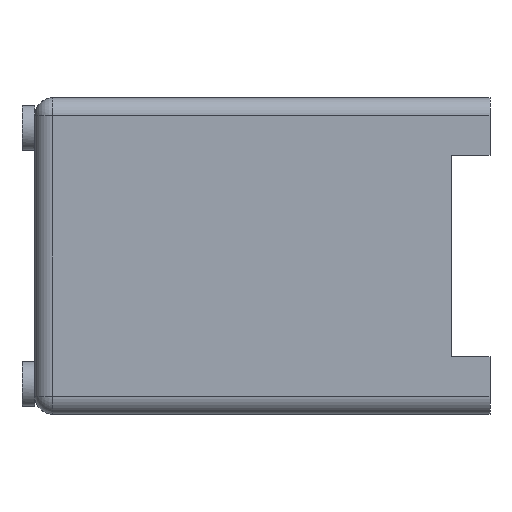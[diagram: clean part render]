
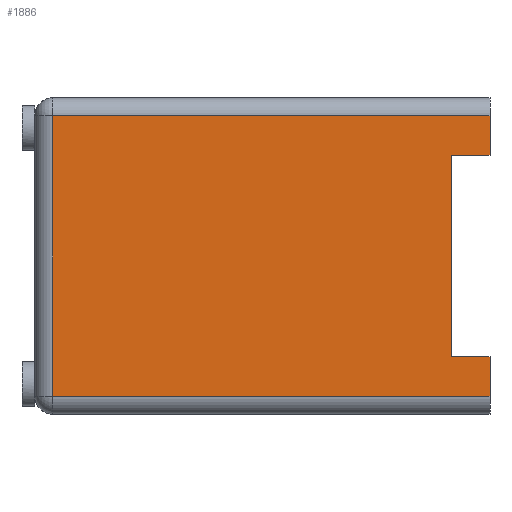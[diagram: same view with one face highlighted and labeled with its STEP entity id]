
A CAD part, left-side view. The second image highlights one B-rep face of the part: STEP entity #1886.
In plain terms, the highlighted planar face has unit normal (-1, 0, 0).
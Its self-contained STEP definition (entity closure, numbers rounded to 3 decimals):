
#4 = EDGE_CURVE ( 'NONE', #798, #2112, #1876, .T. ) ;
#59 = DIRECTION ( 'NONE',  ( 0., 0., 1. ) ) ;
#72 = ORIENTED_EDGE ( 'NONE', *, *, #1344, .T. ) ;
#96 = DIRECTION ( 'NONE',  ( -1., 0., 0. ) ) ;
#103 = CARTESIAN_POINT ( 'NONE',  ( 0., 0., -29.566 ) ) ;
#123 = DIRECTION ( 'NONE',  ( 0., 0., -1. ) ) ;
#158 = ORIENTED_EDGE ( 'NONE', *, *, #684, .T. ) ;
#226 = EDGE_CURVE ( 'NONE', #2142, #892, #342, .T. ) ;
#231 = CARTESIAN_POINT ( 'NONE',  ( 0., 0., -5.69 ) ) ;
#252 = LINE ( 'NONE', #1447, #1040 ) ;
#303 = ORIENTED_EDGE ( 'NONE', *, *, #226, .T. ) ;
#342 = LINE ( 'NONE', #858, #1120 ) ;
#353 = CARTESIAN_POINT ( 'NONE',  ( 0., 43.307, -29.566 ) ) ;
#359 = VERTEX_POINT ( 'NONE', #1167 ) ;
#436 = LINE ( 'NONE', #103, #1429 ) ;
#439 = FACE_OUTER_BOUND ( 'NONE', #701, .T. ) ;
#496 = CARTESIAN_POINT ( 'NONE',  ( 0., 3.81, -5.69 ) ) ;
#515 = DIRECTION ( 'NONE',  ( 0., 0., -1. ) ) ;
#518 = DIRECTION ( 'NONE',  ( 0., 1., 0. ) ) ;
#522 = CARTESIAN_POINT ( 'NONE',  ( 0., 0., -1.778 ) ) ;
#523 = VERTEX_POINT ( 'NONE', #648 ) ;
#631 = DIRECTION ( 'NONE',  ( 0., -1., 0. ) ) ;
#648 = CARTESIAN_POINT ( 'NONE',  ( 0., 0., -29.566 ) ) ;
#657 = EDGE_CURVE ( 'NONE', #1783, #798, #669, .T. ) ;
#659 = CARTESIAN_POINT ( 'NONE',  ( 0., 0., -31.344 ) ) ;
#669 = LINE ( 'NONE', #496, #1096 ) ;
#679 = DIRECTION ( 'NONE',  ( 0., 0., 1. ) ) ;
#684 = EDGE_CURVE ( 'NONE', #523, #359, #1039, .T. ) ;
#698 = DIRECTION ( 'NONE',  ( 0., 1., 0. ) ) ;
#701 = EDGE_LOOP ( 'NONE', ( #2116, #303, #1740, #72, #158, #1464, #1935, #825 ) ) ;
#784 = VECTOR ( 'NONE', #59, 1000. ) ;
#798 = VERTEX_POINT ( 'NONE', #2208 ) ;
#825 = ORIENTED_EDGE ( 'NONE', *, *, #657, .F. ) ;
#854 = EDGE_CURVE ( 'NONE', #892, #2178, #2091, .T. ) ;
#858 = CARTESIAN_POINT ( 'NONE',  ( 0., 45.085, -1.778 ) ) ;
#873 = CARTESIAN_POINT ( 'NONE',  ( 0., 43.307, -1.778 ) ) ;
#892 = VERTEX_POINT ( 'NONE', #873 ) ;
#947 = DIRECTION ( 'NONE',  ( 0., 0., 1. ) ) ;
#989 = LINE ( 'NONE', #1873, #784 ) ;
#1002 = CARTESIAN_POINT ( 'NONE',  ( 0., 3.81, -25.654 ) ) ;
#1039 = LINE ( 'NONE', #659, #1383 ) ;
#1040 = VECTOR ( 'NONE', #631, 1000. ) ;
#1066 = EDGE_CURVE ( 'NONE', #2112, #359, #252, .T. ) ;
#1083 = VECTOR ( 'NONE', #123, 1000. ) ;
#1096 = VECTOR ( 'NONE', #518, 1000. ) ;
#1120 = VECTOR ( 'NONE', #698, 1000. ) ;
#1153 = CARTESIAN_POINT ( 'NONE',  ( 0., 0., -31.344 ) ) ;
#1167 = CARTESIAN_POINT ( 'NONE',  ( 0., 0., -25.654 ) ) ;
#1280 = AXIS2_PLACEMENT_3D ( 'NONE', #1153, #96, #947 ) ;
#1344 = EDGE_CURVE ( 'NONE', #2178, #523, #436, .T. ) ;
#1383 = VECTOR ( 'NONE', #679, 1000. ) ;
#1429 = VECTOR ( 'NONE', #1671, 1000. ) ;
#1447 = CARTESIAN_POINT ( 'NONE',  ( 0., 3.81, -25.654 ) ) ;
#1464 = ORIENTED_EDGE ( 'NONE', *, *, #1066, .F. ) ;
#1472 = PLANE ( 'NONE',  #1280 ) ;
#1575 = VECTOR ( 'NONE', #515, 1000. ) ;
#1596 = EDGE_CURVE ( 'NONE', #1783, #2142, #989, .T. ) ;
#1671 = DIRECTION ( 'NONE',  ( 0., -1., 0. ) ) ;
#1740 = ORIENTED_EDGE ( 'NONE', *, *, #854, .T. ) ;
#1783 = VERTEX_POINT ( 'NONE', #231 ) ;
#1873 = CARTESIAN_POINT ( 'NONE',  ( 0., 0., -31.344 ) ) ;
#1876 = LINE ( 'NONE', #1002, #1083 ) ;
#1886 = ADVANCED_FACE ( 'NONE', ( #439 ), #1472, .T. ) ;
#1894 = CARTESIAN_POINT ( 'NONE',  ( 0., 3.81, -25.654 ) ) ;
#1935 = ORIENTED_EDGE ( 'NONE', *, *, #4, .F. ) ;
#2083 = CARTESIAN_POINT ( 'NONE',  ( 0., 43.307, -31.344 ) ) ;
#2091 = LINE ( 'NONE', #2083, #1575 ) ;
#2112 = VERTEX_POINT ( 'NONE', #1894 ) ;
#2116 = ORIENTED_EDGE ( 'NONE', *, *, #1596, .T. ) ;
#2142 = VERTEX_POINT ( 'NONE', #522 ) ;
#2178 = VERTEX_POINT ( 'NONE', #353 ) ;
#2208 = CARTESIAN_POINT ( 'NONE',  ( 0., 3.81, -5.69 ) ) ;
